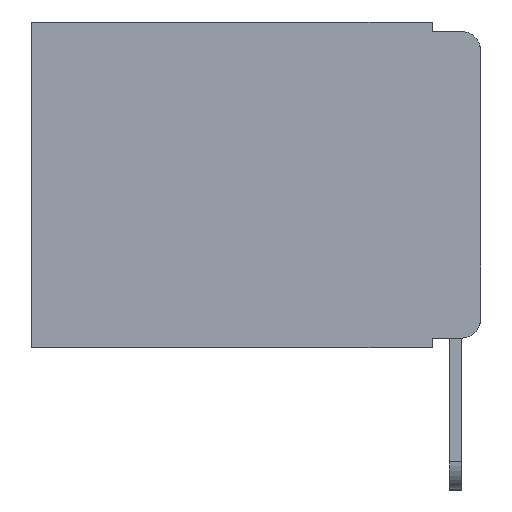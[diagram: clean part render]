
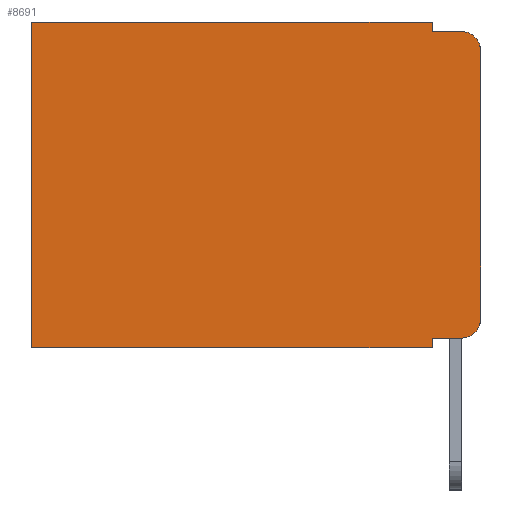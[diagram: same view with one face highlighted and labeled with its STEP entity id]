
A CAD part, left-side view. The second image highlights one B-rep face of the part: STEP entity #8691.
In plain terms, the highlighted planar face has unit normal (-1, 0, 0).
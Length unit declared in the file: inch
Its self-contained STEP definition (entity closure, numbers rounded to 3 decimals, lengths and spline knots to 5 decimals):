
#58 = FACE_OUTER_BOUND ( 'NONE', #9826, .T. ) ;
#114 = DIRECTION ( 'NONE',  ( 0., 0., -1. ) ) ;
#191 = CARTESIAN_POINT ( 'NONE',  ( 0.298, 0.02, -0.03 ) ) ;
#273 = CIRCLE ( 'NONE', #8595, 0.02 ) ;
#411 = DIRECTION ( 'NONE',  ( 0., -1., 0. ) ) ;
#486 = LINE ( 'NONE', #5712, #2102 ) ;
#617 = VECTOR ( 'NONE', #9476, 39.37008 ) ;
#621 = CARTESIAN_POINT ( 'NONE',  ( 0.298, 0.02, -0.01 ) ) ;
#635 = CARTESIAN_POINT ( 'NONE',  ( 0.298, 0.473, 0. ) ) ;
#736 = CARTESIAN_POINT ( 'NONE',  ( 0.298, 0., 0. ) ) ;
#800 = ORIENTED_EDGE ( 'NONE', *, *, #7721, .F. ) ;
#865 = CARTESIAN_POINT ( 'NONE',  ( 0.298, 0.473, -0.343 ) ) ;
#877 = DIRECTION ( 'NONE',  ( 0., -1., 0. ) ) ;
#1188 = VECTOR ( 'NONE', #1597, 39.37008 ) ;
#1199 = EDGE_CURVE ( 'NONE', #9380, #9095, #3797, .T. ) ;
#1458 = CARTESIAN_POINT ( 'NONE',  ( 0.298, 0., -0.313 ) ) ;
#1484 = DIRECTION ( 'NONE',  ( 0., 0., -1. ) ) ;
#1540 = LINE ( 'NONE', #4197, #1188 ) ;
#1597 = DIRECTION ( 'NONE',  ( 0., 0., -1. ) ) ;
#1947 = ORIENTED_EDGE ( 'NONE', *, *, #1199, .T. ) ;
#2102 = VECTOR ( 'NONE', #7265, 39.37008 ) ;
#2116 = VERTEX_POINT ( 'NONE', #4934 ) ;
#2178 = ORIENTED_EDGE ( 'NONE', *, *, #8148, .F. ) ;
#2260 = DIRECTION ( 'NONE',  ( 0., 0., -1. ) ) ;
#2268 = CARTESIAN_POINT ( 'NONE',  ( 0.298, 0.473, 0. ) ) ;
#2366 = DIRECTION ( 'NONE',  ( 1., 0., 0. ) ) ;
#2455 = EDGE_CURVE ( 'NONE', #2116, #4797, #2707, .T. ) ;
#2508 = ORIENTED_EDGE ( 'NONE', *, *, #2455, .F. ) ;
#2707 = LINE ( 'NONE', #6089, #617 ) ;
#2903 = ORIENTED_EDGE ( 'NONE', *, *, #3463, .F. ) ;
#3171 = CARTESIAN_POINT ( 'NONE',  ( 0.298, 0.051, 0. ) ) ;
#3290 = AXIS2_PLACEMENT_3D ( 'NONE', #10236, #3613, #114 ) ;
#3448 = PLANE ( 'NONE',  #6158 ) ;
#3463 = EDGE_CURVE ( 'NONE', #4797, #6112, #3940, .T. ) ;
#3613 = DIRECTION ( 'NONE',  ( -1., 0., 0. ) ) ;
#3689 = DIRECTION ( 'NONE',  ( 0., 0., -1. ) ) ;
#3797 = LINE ( 'NONE', #4747, #7139 ) ;
#3940 = LINE ( 'NONE', #10729, #9622 ) ;
#4030 = VERTEX_POINT ( 'NONE', #865 ) ;
#4197 = CARTESIAN_POINT ( 'NONE',  ( 0.298, 0., 0. ) ) ;
#4359 = VECTOR ( 'NONE', #6719, 39.37008 ) ;
#4747 = CARTESIAN_POINT ( 'NONE',  ( 0.298, 0.051, -0.333 ) ) ;
#4797 = VERTEX_POINT ( 'NONE', #7995 ) ;
#4828 = VERTEX_POINT ( 'NONE', #6162 ) ;
#4901 = DIRECTION ( 'NONE',  ( 0., 1., 0. ) ) ;
#4934 = CARTESIAN_POINT ( 'NONE',  ( 0.298, 0.051, 0. ) ) ;
#5355 = DIRECTION ( 'NONE',  ( -1., 0., 0. ) ) ;
#5712 = CARTESIAN_POINT ( 'NONE',  ( 0.298, 0., -0.343 ) ) ;
#6011 = CARTESIAN_POINT ( 'NONE',  ( 0.298, 0., 0. ) ) ;
#6089 = CARTESIAN_POINT ( 'NONE',  ( 0.298, 0.051, 0. ) ) ;
#6096 = CARTESIAN_POINT ( 'NONE',  ( 0.298, 0., -0.03 ) ) ;
#6112 = VERTEX_POINT ( 'NONE', #621 ) ;
#6158 = AXIS2_PLACEMENT_3D ( 'NONE', #6011, #2366, #2260 ) ;
#6162 = CARTESIAN_POINT ( 'NONE',  ( 0.298, 0.051, -0.343 ) ) ;
#6188 = EDGE_CURVE ( 'NONE', #2116, #6774, #9108, .T. ) ;
#6285 = VECTOR ( 'NONE', #4901, 39.37008 ) ;
#6719 = DIRECTION ( 'NONE',  ( 0., 0., -1. ) ) ;
#6774 = VERTEX_POINT ( 'NONE', #635 ) ;
#6777 = CARTESIAN_POINT ( 'NONE',  ( 0.298, 0.02, -0.333 ) ) ;
#7039 = EDGE_CURVE ( 'NONE', #10921, #6112, #273, .T. ) ;
#7063 = VECTOR ( 'NONE', #1484, 39.37008 ) ;
#7139 = VECTOR ( 'NONE', #411, 39.37008 ) ;
#7265 = DIRECTION ( 'NONE',  ( 0., 1., 0. ) ) ;
#7317 = LINE ( 'NONE', #2268, #7063 ) ;
#7391 = ORIENTED_EDGE ( 'NONE', *, *, #7039, .T. ) ;
#7437 = EDGE_CURVE ( 'NONE', #9095, #8913, #10226, .T. ) ;
#7721 = EDGE_CURVE ( 'NONE', #9380, #4828, #8372, .T. ) ;
#7793 = ORIENTED_EDGE ( 'NONE', *, *, #6188, .T. ) ;
#7995 = CARTESIAN_POINT ( 'NONE',  ( 0.298, 0.051, -0.01 ) ) ;
#8148 = EDGE_CURVE ( 'NONE', #10921, #8913, #1540, .T. ) ;
#8179 = ORIENTED_EDGE ( 'NONE', *, *, #9709, .T. ) ;
#8372 = LINE ( 'NONE', #3171, #4359 ) ;
#8595 = AXIS2_PLACEMENT_3D ( 'NONE', #191, #5355, #3689 ) ;
#8691 = ADVANCED_FACE ( 'NONE', ( #58 ), #3448, .F. ) ;
#8913 = VERTEX_POINT ( 'NONE', #1458 ) ;
#9095 = VERTEX_POINT ( 'NONE', #6777 ) ;
#9108 = LINE ( 'NONE', #736, #6285 ) ;
#9380 = VERTEX_POINT ( 'NONE', #10217 ) ;
#9476 = DIRECTION ( 'NONE',  ( 0., 0., -1. ) ) ;
#9583 = ORIENTED_EDGE ( 'NONE', *, *, #7437, .T. ) ;
#9604 = ORIENTED_EDGE ( 'NONE', *, *, #9700, .F. ) ;
#9622 = VECTOR ( 'NONE', #877, 39.37008 ) ;
#9700 = EDGE_CURVE ( 'NONE', #4828, #4030, #486, .T. ) ;
#9709 = EDGE_CURVE ( 'NONE', #6774, #4030, #7317, .T. ) ;
#9826 = EDGE_LOOP ( 'NONE', ( #2178, #7391, #2903, #2508, #7793, #8179, #9604, #800, #1947, #9583 ) ) ;
#10217 = CARTESIAN_POINT ( 'NONE',  ( 0.298, 0.051, -0.333 ) ) ;
#10226 = CIRCLE ( 'NONE', #3290, 0.02 ) ;
#10236 = CARTESIAN_POINT ( 'NONE',  ( 0.298, 0.02, -0.313 ) ) ;
#10729 = CARTESIAN_POINT ( 'NONE',  ( 0.298, 0.051, -0.01 ) ) ;
#10921 = VERTEX_POINT ( 'NONE', #6096 ) ;
